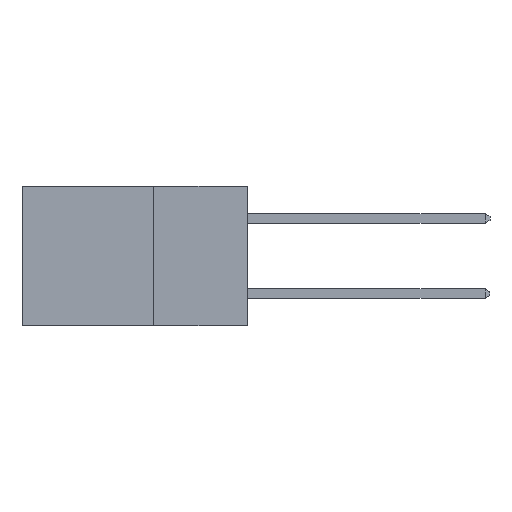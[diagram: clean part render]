
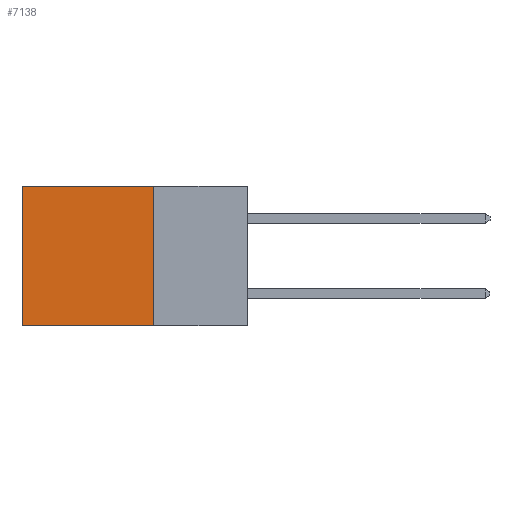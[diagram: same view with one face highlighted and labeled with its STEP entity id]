
A CAD part, left-side view. The second image highlights one B-rep face of the part: STEP entity #7138.
In plain terms, the highlighted planar face has unit normal (-1, 0, 0).
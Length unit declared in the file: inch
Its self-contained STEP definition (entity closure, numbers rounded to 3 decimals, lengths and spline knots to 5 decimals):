
#546 = LINE ( 'NONE', #1817, #14230 ) ;
#738 = LINE ( 'NONE', #11082, #14845 ) ;
#898 = DIRECTION ( 'NONE',  ( 0., 0., -1. ) ) ;
#930 = VECTOR ( 'NONE', #898, 39.37008 ) ;
#1112 = VERTEX_POINT ( 'NONE', #9087 ) ;
#1586 = EDGE_CURVE ( 'NONE', #4502, #1112, #738, .T. ) ;
#1817 = CARTESIAN_POINT ( 'NONE',  ( 0.298, 0.6, 0. ) ) ;
#2350 = CARTESIAN_POINT ( 'NONE',  ( 0.298, 0.25, -0.37 ) ) ;
#2477 = DIRECTION ( 'NONE',  ( 0., 1., 0. ) ) ;
#3176 = AXIS2_PLACEMENT_3D ( 'NONE', #7510, #11460, #10171 ) ;
#3418 = VECTOR ( 'NONE', #2477, 39.37008 ) ;
#3526 = EDGE_CURVE ( 'NONE', #4524, #8592, #10054, .T. ) ;
#3594 = CARTESIAN_POINT ( 'NONE',  ( 0.298, 0.25, -0.37 ) ) ;
#4502 = VERTEX_POINT ( 'NONE', #16591 ) ;
#4524 = VERTEX_POINT ( 'NONE', #3594 ) ;
#4931 = LINE ( 'NONE', #7523, #930 ) ;
#5697 = ORIENTED_EDGE ( 'NONE', *, *, #8880, .F. ) ;
#5774 = EDGE_LOOP ( 'NONE', ( #16691, #7749, #5697, #7810 ) ) ;
#7138 = ADVANCED_FACE ( 'NONE', ( #16010 ), #8883, .F. ) ;
#7510 = CARTESIAN_POINT ( 'NONE',  ( 0.298, 0.25, 0. ) ) ;
#7523 = CARTESIAN_POINT ( 'NONE',  ( 0.298, 0.25, 0. ) ) ;
#7749 = ORIENTED_EDGE ( 'NONE', *, *, #3526, .F. ) ;
#7810 = ORIENTED_EDGE ( 'NONE', *, *, #1586, .T. ) ;
#7946 = EDGE_CURVE ( 'NONE', #1112, #8592, #546, .T. ) ;
#8589 = DIRECTION ( 'NONE',  ( 0., 1., 0. ) ) ;
#8592 = VERTEX_POINT ( 'NONE', #9708 ) ;
#8880 = EDGE_CURVE ( 'NONE', #4502, #4524, #4931, .T. ) ;
#8883 = PLANE ( 'NONE',  #3176 ) ;
#9087 = CARTESIAN_POINT ( 'NONE',  ( 0.298, 0.6, 0. ) ) ;
#9708 = CARTESIAN_POINT ( 'NONE',  ( 0.298, 0.6, -0.37 ) ) ;
#9779 = DIRECTION ( 'NONE',  ( 0., 0., -1. ) ) ;
#10054 = LINE ( 'NONE', #2350, #3418 ) ;
#10171 = DIRECTION ( 'NONE',  ( 0., 0., -1. ) ) ;
#11082 = CARTESIAN_POINT ( 'NONE',  ( 0.298, 0.25, 0. ) ) ;
#11460 = DIRECTION ( 'NONE',  ( 1., 0., 0. ) ) ;
#14230 = VECTOR ( 'NONE', #9779, 39.37008 ) ;
#14845 = VECTOR ( 'NONE', #8589, 39.37008 ) ;
#16010 = FACE_OUTER_BOUND ( 'NONE', #5774, .T. ) ;
#16591 = CARTESIAN_POINT ( 'NONE',  ( 0.298, 0.25, 0. ) ) ;
#16691 = ORIENTED_EDGE ( 'NONE', *, *, #7946, .T. ) ;
